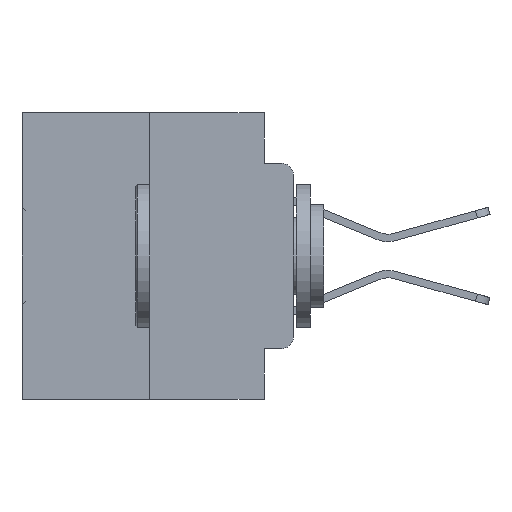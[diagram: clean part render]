
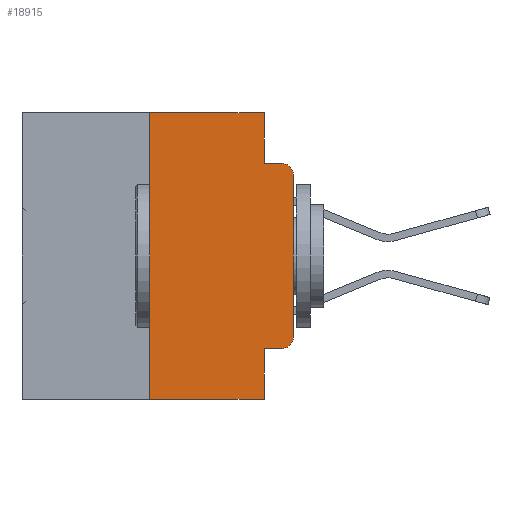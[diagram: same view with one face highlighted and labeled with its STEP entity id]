
A CAD part, left-side view. The second image highlights one B-rep face of the part: STEP entity #18915.
In plain terms, the highlighted planar face has unit normal (-1, 0, 0).
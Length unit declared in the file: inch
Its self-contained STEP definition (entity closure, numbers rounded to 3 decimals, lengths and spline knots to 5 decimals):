
#109 = CARTESIAN_POINT ( 'NONE',  ( 0., 0.25, 0. ) ) ;
#197 = CARTESIAN_POINT ( 'NONE',  ( 0., 0.473, -0.5 ) ) ;
#649 = LINE ( 'NONE', #3937, #28128 ) ;
#1423 = EDGE_CURVE ( 'NONE', #31527, #18584, #17190, .T. ) ;
#1636 = EDGE_CURVE ( 'NONE', #12656, #3953, #11342, .T. ) ;
#1937 = EDGE_CURVE ( 'NONE', #3953, #3469, #22504, .T. ) ;
#2013 = ORIENTED_EDGE ( 'NONE', *, *, #28261, .T. ) ;
#2657 = AXIS2_PLACEMENT_3D ( 'NONE', #21973, #6019, #24581 ) ;
#2759 = CARTESIAN_POINT ( 'NONE',  ( 0., 0.25, 0. ) ) ;
#3469 = VERTEX_POINT ( 'NONE', #17412 ) ;
#3937 = CARTESIAN_POINT ( 'NONE',  ( 0., 0.051, -0.4115 ) ) ;
#3953 = VERTEX_POINT ( 'NONE', #28200 ) ;
#4003 = FACE_OUTER_BOUND ( 'NONE', #4251, .T. ) ;
#4251 = EDGE_LOOP ( 'NONE', ( #19617, #15069, #16760, #30629, #12151, #20842, #2013, #31034, #10904, #26606 ) ) ;
#4323 = DIRECTION ( 'NONE',  ( -1., 0., 0. ) ) ;
#4581 = CARTESIAN_POINT ( 'NONE',  ( 0., 0.02, -0.3915 ) ) ;
#4932 = VERTEX_POINT ( 'NONE', #13770 ) ;
#6003 = LINE ( 'NONE', #24305, #33978 ) ;
#6019 = DIRECTION ( 'NONE',  ( 1., 0., 0. ) ) ;
#6729 = CARTESIAN_POINT ( 'NONE',  ( 0., 0.051, -0.0885 ) ) ;
#7232 = CARTESIAN_POINT ( 'NONE',  ( 0., 0.02, -0.0885 ) ) ;
#7386 = VERTEX_POINT ( 'NONE', #26402 ) ;
#7417 = CIRCLE ( 'NONE', #32280, 0.02 ) ;
#8618 = CARTESIAN_POINT ( 'NONE',  ( 0., 0.02, -0.4115 ) ) ;
#8770 = DIRECTION ( 'NONE',  ( 0., 0., 1. ) ) ;
#8935 = DIRECTION ( 'NONE',  ( 0., -1., 0. ) ) ;
#8957 = VECTOR ( 'NONE', #8935, 39.37008 ) ;
#10695 = LINE ( 'NONE', #2759, #16966 ) ;
#10904 = ORIENTED_EDGE ( 'NONE', *, *, #32678, .T. ) ;
#11342 = CIRCLE ( 'NONE', #16550, 0.02 ) ;
#11515 = VERTEX_POINT ( 'NONE', #19266 ) ;
#11977 = DIRECTION ( 'NONE',  ( 0., 0., -1. ) ) ;
#12119 = DIRECTION ( 'NONE',  ( -1., 0., 0. ) ) ;
#12151 = ORIENTED_EDGE ( 'NONE', *, *, #26974, .F. ) ;
#12656 = VERTEX_POINT ( 'NONE', #8618 ) ;
#13770 = CARTESIAN_POINT ( 'NONE',  ( 0., 0.051, -0.4115 ) ) ;
#13963 = DIRECTION ( 'NONE',  ( 0., 0., -1. ) ) ;
#15069 = ORIENTED_EDGE ( 'NONE', *, *, #33337, .T. ) ;
#16550 = AXIS2_PLACEMENT_3D ( 'NONE', #4581, #4323, #11977 ) ;
#16580 = PLANE ( 'NONE',  #2657 ) ;
#16760 = ORIENTED_EDGE ( 'NONE', *, *, #1423, .F. ) ;
#16966 = VECTOR ( 'NONE', #24084, 39.37008 ) ;
#17190 = LINE ( 'NONE', #26792, #31872 ) ;
#17245 = VECTOR ( 'NONE', #24250, 39.37008 ) ;
#17412 = CARTESIAN_POINT ( 'NONE',  ( 0., 0., -0.1085 ) ) ;
#18055 = LINE ( 'NONE', #197, #17245 ) ;
#18584 = VERTEX_POINT ( 'NONE', #7232 ) ;
#18915 = ADVANCED_FACE ( 'NONE', ( #4003 ), #16580, .F. ) ;
#19045 = DIRECTION ( 'NONE',  ( 0., 0., -1. ) ) ;
#19266 = CARTESIAN_POINT ( 'NONE',  ( 0., 0.25, -0.5 ) ) ;
#19569 = DIRECTION ( 'NONE',  ( 0., -1., 0. ) ) ;
#19617 = ORIENTED_EDGE ( 'NONE', *, *, #1937, .T. ) ;
#20296 = EDGE_CURVE ( 'NONE', #11515, #29534, #10695, .T. ) ;
#20376 = CARTESIAN_POINT ( 'NONE',  ( 0., 0., 0. ) ) ;
#20487 = VERTEX_POINT ( 'NONE', #22270 ) ;
#20672 = VECTOR ( 'NONE', #13963, 39.37008 ) ;
#20842 = ORIENTED_EDGE ( 'NONE', *, *, #20296, .F. ) ;
#21973 = CARTESIAN_POINT ( 'NONE',  ( 0., 0.473, 0. ) ) ;
#22270 = CARTESIAN_POINT ( 'NONE',  ( 0., 0.051, -0.5 ) ) ;
#22504 = LINE ( 'NONE', #20376, #29429 ) ;
#24084 = DIRECTION ( 'NONE',  ( 0., 0., 1. ) ) ;
#24250 = DIRECTION ( 'NONE',  ( 0., -1., 0. ) ) ;
#24305 = CARTESIAN_POINT ( 'NONE',  ( 0., 0.051, 0. ) ) ;
#24445 = CARTESIAN_POINT ( 'NONE',  ( 0., 0.051, 0. ) ) ;
#24581 = DIRECTION ( 'NONE',  ( 0., 0., -1. ) ) ;
#26402 = CARTESIAN_POINT ( 'NONE',  ( 0., 0.051, 0. ) ) ;
#26606 = ORIENTED_EDGE ( 'NONE', *, *, #1636, .T. ) ;
#26792 = CARTESIAN_POINT ( 'NONE',  ( 0., 0.051, -0.0885 ) ) ;
#26878 = EDGE_CURVE ( 'NONE', #7386, #31527, #6003, .T. ) ;
#26974 = EDGE_CURVE ( 'NONE', #29534, #7386, #29165, .T. ) ;
#27655 = LINE ( 'NONE', #24445, #20672 ) ;
#27823 = DIRECTION ( 'NONE',  ( 0., -1., 0. ) ) ;
#27896 = CARTESIAN_POINT ( 'NONE',  ( 0., 0.02, -0.1085 ) ) ;
#28128 = VECTOR ( 'NONE', #27823, 39.37008 ) ;
#28200 = CARTESIAN_POINT ( 'NONE',  ( 0., 0., -0.3915 ) ) ;
#28261 = EDGE_CURVE ( 'NONE', #11515, #20487, #18055, .T. ) ;
#29165 = LINE ( 'NONE', #32591, #8957 ) ;
#29429 = VECTOR ( 'NONE', #8770, 39.37008 ) ;
#29534 = VERTEX_POINT ( 'NONE', #109 ) ;
#30496 = DIRECTION ( 'NONE',  ( 0., 0., -1. ) ) ;
#30629 = ORIENTED_EDGE ( 'NONE', *, *, #26878, .F. ) ;
#31034 = ORIENTED_EDGE ( 'NONE', *, *, #33769, .F. ) ;
#31527 = VERTEX_POINT ( 'NONE', #6729 ) ;
#31872 = VECTOR ( 'NONE', #19569, 39.37008 ) ;
#32280 = AXIS2_PLACEMENT_3D ( 'NONE', #27896, #12119, #30496 ) ;
#32591 = CARTESIAN_POINT ( 'NONE',  ( 0., 0.473, 0. ) ) ;
#32678 = EDGE_CURVE ( 'NONE', #4932, #12656, #649, .T. ) ;
#33337 = EDGE_CURVE ( 'NONE', #3469, #18584, #7417, .T. ) ;
#33769 = EDGE_CURVE ( 'NONE', #4932, #20487, #27655, .T. ) ;
#33978 = VECTOR ( 'NONE', #19045, 39.37008 ) ;
